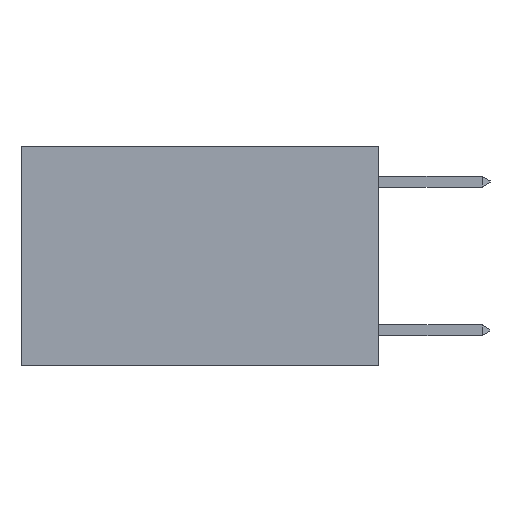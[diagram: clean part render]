
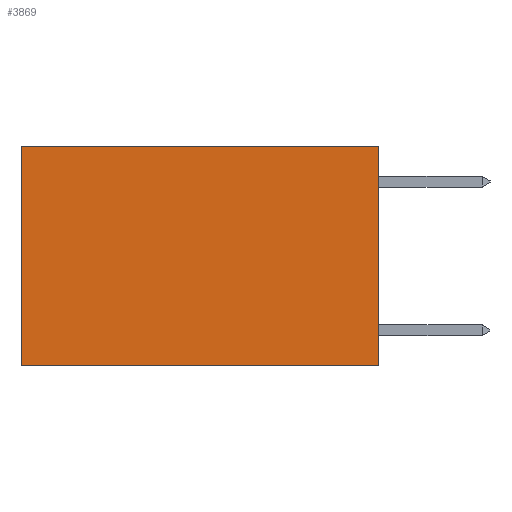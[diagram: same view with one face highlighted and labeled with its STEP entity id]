
A CAD part, left-side view. The second image highlights one B-rep face of the part: STEP entity #3869.
In plain terms, the highlighted planar face has unit normal (-1, 0, 0).
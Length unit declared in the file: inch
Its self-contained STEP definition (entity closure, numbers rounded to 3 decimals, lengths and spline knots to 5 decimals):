
#215 = CARTESIAN_POINT ( 'NONE',  ( 0.2625, 0., 0. ) ) ;
#449 = DIRECTION ( 'NONE',  ( 0., 0., -1. ) ) ;
#501 = DIRECTION ( 'NONE',  ( 0., 1., 0. ) ) ;
#590 = VERTEX_POINT ( 'NONE', #5569 ) ;
#621 = EDGE_CURVE ( 'NONE', #4862, #5877, #3826, .T. ) ;
#642 = ORIENTED_EDGE ( 'NONE', *, *, #4113, .T. ) ;
#2142 = DIRECTION ( 'NONE',  ( 0., 0., -1. ) ) ;
#2360 = EDGE_CURVE ( 'NONE', #3786, #4862, #4211, .T. ) ;
#2530 = VECTOR ( 'NONE', #449, 39.37008 ) ;
#2804 = LINE ( 'NONE', #4168, #4289 ) ;
#2877 = CARTESIAN_POINT ( 'NONE',  ( 0.2625, 0.6, -0.37 ) ) ;
#2893 = DIRECTION ( 'NONE',  ( 0., 1., 0. ) ) ;
#3149 = LINE ( 'NONE', #3768, #4835 ) ;
#3164 = EDGE_LOOP ( 'NONE', ( #642, #6481, #6770, #6951 ) ) ;
#3248 = FACE_OUTER_BOUND ( 'NONE', #3164, .T. ) ;
#3668 = CARTESIAN_POINT ( 'NONE',  ( 0.2625, 0., -0.37 ) ) ;
#3768 = CARTESIAN_POINT ( 'NONE',  ( 0.2625, 0.6, 0. ) ) ;
#3786 = VERTEX_POINT ( 'NONE', #7690 ) ;
#3826 = LINE ( 'NONE', #3668, #6954 ) ;
#3869 = ADVANCED_FACE ( 'NONE', ( #3248 ), #4660, .F. ) ;
#4113 = EDGE_CURVE ( 'NONE', #590, #5877, #3149, .T. ) ;
#4168 = CARTESIAN_POINT ( 'NONE',  ( 0.2625, 0., 0. ) ) ;
#4211 = LINE ( 'NONE', #7360, #2530 ) ;
#4289 = VECTOR ( 'NONE', #2893, 39.37008 ) ;
#4660 = PLANE ( 'NONE',  #6041 ) ;
#4835 = VECTOR ( 'NONE', #6882, 39.37008 ) ;
#4862 = VERTEX_POINT ( 'NONE', #5126 ) ;
#5126 = CARTESIAN_POINT ( 'NONE',  ( 0.2625, 0., -0.37 ) ) ;
#5569 = CARTESIAN_POINT ( 'NONE',  ( 0.2625, 0.6, 0. ) ) ;
#5877 = VERTEX_POINT ( 'NONE', #2877 ) ;
#5940 = DIRECTION ( 'NONE',  ( 1., 0., 0. ) ) ;
#6041 = AXIS2_PLACEMENT_3D ( 'NONE', #215, #5940, #2142 ) ;
#6481 = ORIENTED_EDGE ( 'NONE', *, *, #621, .F. ) ;
#6770 = ORIENTED_EDGE ( 'NONE', *, *, #2360, .F. ) ;
#6882 = DIRECTION ( 'NONE',  ( 0., 0., -1. ) ) ;
#6951 = ORIENTED_EDGE ( 'NONE', *, *, #7191, .T. ) ;
#6954 = VECTOR ( 'NONE', #501, 39.37008 ) ;
#7191 = EDGE_CURVE ( 'NONE', #3786, #590, #2804, .T. ) ;
#7360 = CARTESIAN_POINT ( 'NONE',  ( 0.2625, 0., 0. ) ) ;
#7690 = CARTESIAN_POINT ( 'NONE',  ( 0.2625, 0., 0. ) ) ;
